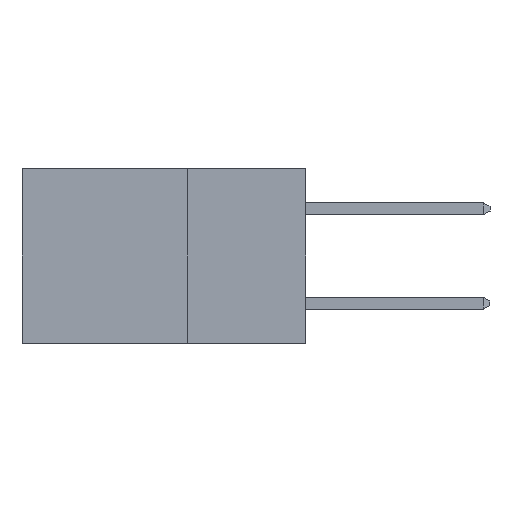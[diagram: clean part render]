
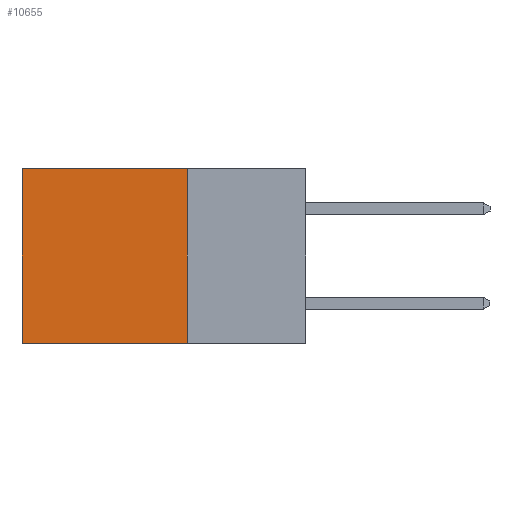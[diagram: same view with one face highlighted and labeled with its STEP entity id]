
A CAD part, left-side view. The second image highlights one B-rep face of the part: STEP entity #10655.
In plain terms, the highlighted planar face has unit normal (-1, 0, 0).
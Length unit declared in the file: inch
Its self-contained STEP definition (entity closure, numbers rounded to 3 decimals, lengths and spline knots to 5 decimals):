
#201 = VERTEX_POINT ( 'NONE', #5665 ) ;
#352 = EDGE_LOOP ( 'NONE', ( #6166, #8719, #5808, #17099 ) ) ;
#466 = CARTESIAN_POINT ( 'NONE',  ( 0.298, 0.6, -0.37 ) ) ;
#603 = LINE ( 'NONE', #14938, #3731 ) ;
#2645 = VECTOR ( 'NONE', #8478, 39.37008 ) ;
#3251 = CARTESIAN_POINT ( 'NONE',  ( 0.298, 0.6, 0. ) ) ;
#3731 = VECTOR ( 'NONE', #7715, 39.37008 ) ;
#3746 = VERTEX_POINT ( 'NONE', #3251 ) ;
#4830 = EDGE_CURVE ( 'NONE', #15099, #201, #14512, .T. ) ;
#5646 = PLANE ( 'NONE',  #8014 ) ;
#5665 = CARTESIAN_POINT ( 'NONE',  ( 0.298, 0.25, -0.37 ) ) ;
#5808 = ORIENTED_EDGE ( 'NONE', *, *, #4830, .F. ) ;
#6166 = ORIENTED_EDGE ( 'NONE', *, *, #11408, .T. ) ;
#6203 = EDGE_CURVE ( 'NONE', #15099, #3746, #603, .T. ) ;
#7299 = FACE_OUTER_BOUND ( 'NONE', #352, .T. ) ;
#7715 = DIRECTION ( 'NONE',  ( 0., 1., 0. ) ) ;
#8014 = AXIS2_PLACEMENT_3D ( 'NONE', #14866, #9598, #16173 ) ;
#8478 = DIRECTION ( 'NONE',  ( 0., 0., -1. ) ) ;
#8719 = ORIENTED_EDGE ( 'NONE', *, *, #12868, .F. ) ;
#9598 = DIRECTION ( 'NONE',  ( 1., 0., 0. ) ) ;
#10655 = ADVANCED_FACE ( 'NONE', ( #7299 ), #5646, .F. ) ;
#11408 = EDGE_CURVE ( 'NONE', #3746, #14910, #13159, .T. ) ;
#11696 = LINE ( 'NONE', #13757, #14811 ) ;
#12505 = DIRECTION ( 'NONE',  ( 0., 1., 0. ) ) ;
#12868 = EDGE_CURVE ( 'NONE', #201, #14910, #11696, .T. ) ;
#13159 = LINE ( 'NONE', #15027, #2645 ) ;
#13757 = CARTESIAN_POINT ( 'NONE',  ( 0.298, 0.25, -0.37 ) ) ;
#14082 = VECTOR ( 'NONE', #15352, 39.37008 ) ;
#14512 = LINE ( 'NONE', #16791, #14082 ) ;
#14811 = VECTOR ( 'NONE', #12505, 39.37008 ) ;
#14866 = CARTESIAN_POINT ( 'NONE',  ( 0.298, 0.25, 0. ) ) ;
#14910 = VERTEX_POINT ( 'NONE', #466 ) ;
#14938 = CARTESIAN_POINT ( 'NONE',  ( 0.298, 0.25, 0. ) ) ;
#15027 = CARTESIAN_POINT ( 'NONE',  ( 0.298, 0.6, 0. ) ) ;
#15099 = VERTEX_POINT ( 'NONE', #16707 ) ;
#15352 = DIRECTION ( 'NONE',  ( 0., 0., -1. ) ) ;
#16173 = DIRECTION ( 'NONE',  ( 0., 0., -1. ) ) ;
#16707 = CARTESIAN_POINT ( 'NONE',  ( 0.298, 0.25, 0. ) ) ;
#16791 = CARTESIAN_POINT ( 'NONE',  ( 0.298, 0.25, 0. ) ) ;
#17099 = ORIENTED_EDGE ( 'NONE', *, *, #6203, .T. ) ;
